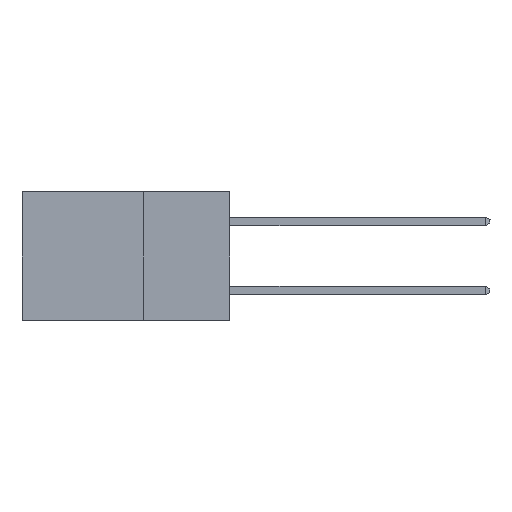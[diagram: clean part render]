
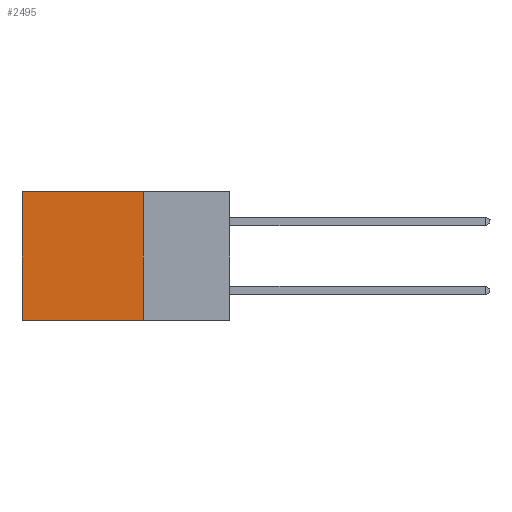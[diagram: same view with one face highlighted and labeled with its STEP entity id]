
A CAD part, left-side view. The second image highlights one B-rep face of the part: STEP entity #2495.
In plain terms, the highlighted planar face has unit normal (-1, 0, 0).
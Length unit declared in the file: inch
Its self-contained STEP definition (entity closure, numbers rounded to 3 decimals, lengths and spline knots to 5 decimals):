
#1411 = ORIENTED_EDGE ( 'NONE', *, *, #3741, .T. ) ;
#1893 = CARTESIAN_POINT ( 'NONE',  ( 0.2615, 0.6, -0.37 ) ) ;
#2209 = CARTESIAN_POINT ( 'NONE',  ( 0.2615, 0.25, -0.37 ) ) ;
#2495 = ADVANCED_FACE ( 'NONE', ( #7461 ), #3654, .F. ) ;
#2775 = AXIS2_PLACEMENT_3D ( 'NONE', #2209, #6204, #7382 ) ;
#3401 = EDGE_CURVE ( 'NONE', #9917, #8120, #10905, .T. ) ;
#3636 = CARTESIAN_POINT ( 'NONE',  ( 0.2615, 0.6, -0.37 ) ) ;
#3654 = PLANE ( 'NONE',  #2775 ) ;
#3741 = EDGE_CURVE ( 'NONE', #8867, #8120, #12485, .T. ) ;
#4133 = CARTESIAN_POINT ( 'NONE',  ( 0.2615, 0.25, -0.37 ) ) ;
#4148 = VECTOR ( 'NONE', #15022, 39.37008 ) ;
#4200 = LINE ( 'NONE', #9388, #8788 ) ;
#4349 = ORIENTED_EDGE ( 'NONE', *, *, #5625, .T. ) ;
#5015 = LINE ( 'NONE', #14070, #11589 ) ;
#5625 = EDGE_CURVE ( 'NONE', #9555, #8867, #4200, .T. ) ;
#6204 = DIRECTION ( 'NONE',  ( 1., 0., 0. ) ) ;
#6375 = DIRECTION ( 'NONE',  ( 0., 0., -1. ) ) ;
#7382 = DIRECTION ( 'NONE',  ( 0., 0., -1. ) ) ;
#7461 = FACE_OUTER_BOUND ( 'NONE', #15364, .T. ) ;
#8120 = VERTEX_POINT ( 'NONE', #3636 ) ;
#8385 = DIRECTION ( 'NONE',  ( 0., 1., 0. ) ) ;
#8639 = EDGE_CURVE ( 'NONE', #9555, #9917, #5015, .T. ) ;
#8788 = VECTOR ( 'NONE', #8385, 39.37008 ) ;
#8867 = VERTEX_POINT ( 'NONE', #10850 ) ;
#9038 = VECTOR ( 'NONE', #13583, 39.37008 ) ;
#9256 = CARTESIAN_POINT ( 'NONE',  ( 0.2615, 0.25, 0. ) ) ;
#9388 = CARTESIAN_POINT ( 'NONE',  ( 0.2615, 0.25, 0. ) ) ;
#9555 = VERTEX_POINT ( 'NONE', #9256 ) ;
#9917 = VERTEX_POINT ( 'NONE', #4133 ) ;
#10850 = CARTESIAN_POINT ( 'NONE',  ( 0.2615, 0.6, 0. ) ) ;
#10905 = LINE ( 'NONE', #13517, #4148 ) ;
#11589 = VECTOR ( 'NONE', #6375, 39.37008 ) ;
#12485 = LINE ( 'NONE', #1893, #9038 ) ;
#13517 = CARTESIAN_POINT ( 'NONE',  ( 0.2615, 0.25, -0.37 ) ) ;
#13583 = DIRECTION ( 'NONE',  ( 0., 0., -1. ) ) ;
#13827 = ORIENTED_EDGE ( 'NONE', *, *, #8639, .F. ) ;
#14070 = CARTESIAN_POINT ( 'NONE',  ( 0.2615, 0.25, -0.37 ) ) ;
#14496 = ORIENTED_EDGE ( 'NONE', *, *, #3401, .F. ) ;
#15022 = DIRECTION ( 'NONE',  ( 0., 1., 0. ) ) ;
#15364 = EDGE_LOOP ( 'NONE', ( #1411, #14496, #13827, #4349 ) ) ;
